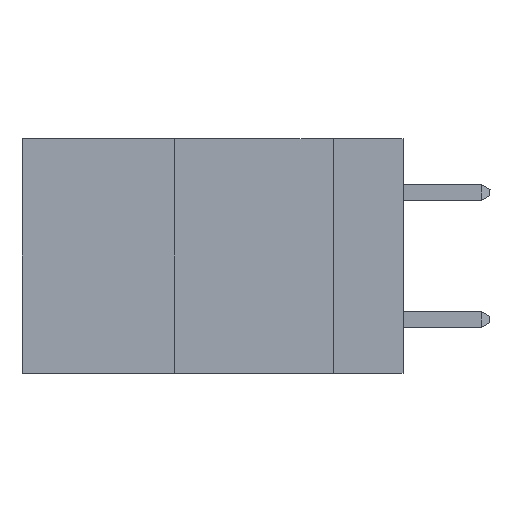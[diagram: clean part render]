
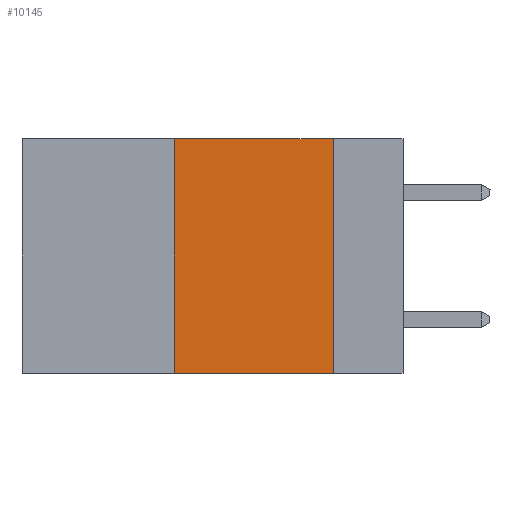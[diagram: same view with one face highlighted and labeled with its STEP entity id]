
A CAD part, left-side view. The second image highlights one B-rep face of the part: STEP entity #10145.
In plain terms, the highlighted planar face has unit normal (-1, 0, 0).
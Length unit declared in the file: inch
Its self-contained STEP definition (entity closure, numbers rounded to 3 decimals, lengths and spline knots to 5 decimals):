
#4 = VERTEX_POINT ( 'NONE', #9795 ) ;
#181 = VERTEX_POINT ( 'NONE', #274 ) ;
#262 = ORIENTED_EDGE ( 'NONE', *, *, #8168, .F. ) ;
#274 = CARTESIAN_POINT ( 'NONE',  ( 0., 0.11, -0.37 ) ) ;
#276 = CARTESIAN_POINT ( 'NONE',  ( 0., 0.6, 0. ) ) ;
#545 = ORIENTED_EDGE ( 'NONE', *, *, #4328, .F. ) ;
#2276 = PLANE ( 'NONE',  #11326 ) ;
#2603 = CARTESIAN_POINT ( 'NONE',  ( 0., 0.6, -0.37 ) ) ;
#2605 = DIRECTION ( 'NONE',  ( 0., -1., 0. ) ) ;
#3001 = EDGE_CURVE ( 'NONE', #4, #181, #6884, .T. ) ;
#3224 = DIRECTION ( 'NONE',  ( 1., 0., 0. ) ) ;
#3365 = CARTESIAN_POINT ( 'NONE',  ( 0., 0.11, 0. ) ) ;
#3548 = EDGE_CURVE ( 'NONE', #7730, #181, #8679, .T. ) ;
#3586 = ORIENTED_EDGE ( 'NONE', *, *, #3548, .F. ) ;
#3595 = DIRECTION ( 'NONE',  ( 0., 0., -1. ) ) ;
#4148 = ORIENTED_EDGE ( 'NONE', *, *, #3001, .T. ) ;
#4327 = VECTOR ( 'NONE', #7416, 39.37008 ) ;
#4328 = EDGE_CURVE ( 'NONE', #4, #7867, #11513, .T. ) ;
#4949 = CARTESIAN_POINT ( 'NONE',  ( 0., 0.36, 0. ) ) ;
#5400 = CARTESIAN_POINT ( 'NONE',  ( 0., 0.6, 0. ) ) ;
#5756 = LINE ( 'NONE', #5400, #7550 ) ;
#6802 = CARTESIAN_POINT ( 'NONE',  ( 0., 0.36, 0. ) ) ;
#6884 = LINE ( 'NONE', #2603, #8955 ) ;
#7097 = EDGE_LOOP ( 'NONE', ( #3586, #262, #545, #4148 ) ) ;
#7416 = DIRECTION ( 'NONE',  ( 0., 0., 1. ) ) ;
#7550 = VECTOR ( 'NONE', #8964, 39.37008 ) ;
#7730 = VERTEX_POINT ( 'NONE', #9172 ) ;
#7867 = VERTEX_POINT ( 'NONE', #4949 ) ;
#8168 = EDGE_CURVE ( 'NONE', #7867, #7730, #5756, .T. ) ;
#8679 = LINE ( 'NONE', #3365, #10424 ) ;
#8955 = VECTOR ( 'NONE', #2605, 39.37008 ) ;
#8964 = DIRECTION ( 'NONE',  ( 0., -1., 0. ) ) ;
#9172 = CARTESIAN_POINT ( 'NONE',  ( 0., 0.11, 0. ) ) ;
#9531 = DIRECTION ( 'NONE',  ( 0., 0., -1. ) ) ;
#9795 = CARTESIAN_POINT ( 'NONE',  ( 0., 0.36, -0.37 ) ) ;
#10145 = ADVANCED_FACE ( 'NONE', ( #10762 ), #2276, .F. ) ;
#10424 = VECTOR ( 'NONE', #3595, 39.37008 ) ;
#10762 = FACE_OUTER_BOUND ( 'NONE', #7097, .T. ) ;
#11326 = AXIS2_PLACEMENT_3D ( 'NONE', #276, #3224, #9531 ) ;
#11513 = LINE ( 'NONE', #6802, #4327 ) ;
